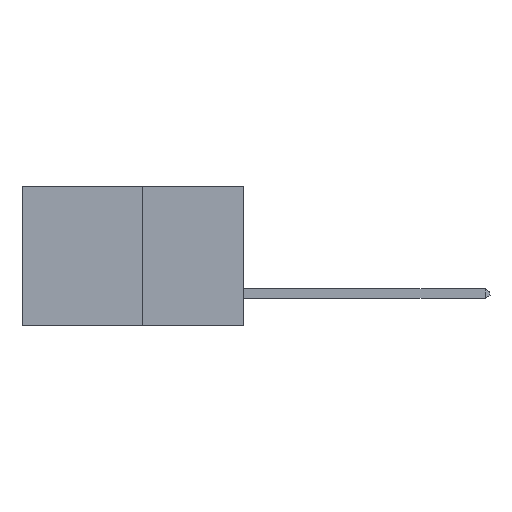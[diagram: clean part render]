
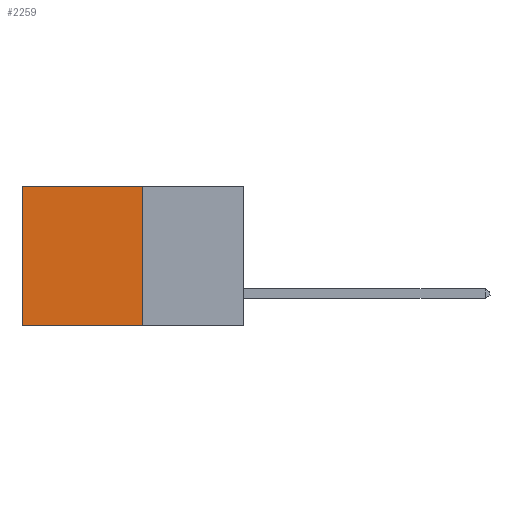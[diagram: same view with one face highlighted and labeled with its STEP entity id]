
A CAD part, left-side view. The second image highlights one B-rep face of the part: STEP entity #2259.
In plain terms, the highlighted planar face has unit normal (-1, 0, 0).
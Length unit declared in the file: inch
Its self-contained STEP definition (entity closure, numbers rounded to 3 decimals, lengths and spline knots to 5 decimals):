
#168 = LINE ( 'NONE', #9690, #10911 ) ;
#216 = VERTEX_POINT ( 'NONE', #3422 ) ;
#265 = EDGE_CURVE ( 'NONE', #3902, #216, #9860, .T. ) ;
#288 = ORIENTED_EDGE ( 'NONE', *, *, #2678, .F. ) ;
#728 = CARTESIAN_POINT ( 'NONE',  ( 0.277, 0.27, -0.37 ) ) ;
#844 = ORIENTED_EDGE ( 'NONE', *, *, #265, .T. ) ;
#880 = DIRECTION ( 'NONE',  ( 0., 1., 0. ) ) ;
#1134 = EDGE_LOOP ( 'NONE', ( #844, #288, #4003, #7695 ) ) ;
#2259 = ADVANCED_FACE ( 'NONE', ( #6381 ), #5868, .F. ) ;
#2678 = EDGE_CURVE ( 'NONE', #2979, #216, #9930, .T. ) ;
#2979 = VERTEX_POINT ( 'NONE', #10078 ) ;
#3100 = VECTOR ( 'NONE', #10730, 39.37008 ) ;
#3422 = CARTESIAN_POINT ( 'NONE',  ( 0.277, 0.59, -0.37 ) ) ;
#3902 = VERTEX_POINT ( 'NONE', #10510 ) ;
#4003 = ORIENTED_EDGE ( 'NONE', *, *, #7244, .F. ) ;
#4107 = VERTEX_POINT ( 'NONE', #10610 ) ;
#5145 = EDGE_CURVE ( 'NONE', #4107, #3902, #7676, .T. ) ;
#5452 = VECTOR ( 'NONE', #8115, 39.37008 ) ;
#5540 = CARTESIAN_POINT ( 'NONE',  ( 0.277, 0.59, -0.37 ) ) ;
#5576 = DIRECTION ( 'NONE',  ( 0., 0., -1. ) ) ;
#5814 = VECTOR ( 'NONE', #880, 39.37008 ) ;
#5868 = PLANE ( 'NONE',  #9458 ) ;
#6083 = CARTESIAN_POINT ( 'NONE',  ( 0.277, 0.27, -0.37 ) ) ;
#6155 = DIRECTION ( 'NONE',  ( 1., 0., 0. ) ) ;
#6381 = FACE_OUTER_BOUND ( 'NONE', #1134, .T. ) ;
#7244 = EDGE_CURVE ( 'NONE', #4107, #2979, #168, .T. ) ;
#7676 = LINE ( 'NONE', #10740, #3100 ) ;
#7695 = ORIENTED_EDGE ( 'NONE', *, *, #5145, .T. ) ;
#8003 = DIRECTION ( 'NONE',  ( 0., 0., -1. ) ) ;
#8115 = DIRECTION ( 'NONE',  ( 0., 0., -1. ) ) ;
#9458 = AXIS2_PLACEMENT_3D ( 'NONE', #6083, #6155, #8003 ) ;
#9690 = CARTESIAN_POINT ( 'NONE',  ( 0.277, 0.27, -0.37 ) ) ;
#9860 = LINE ( 'NONE', #5540, #5452 ) ;
#9930 = LINE ( 'NONE', #728, #5814 ) ;
#10078 = CARTESIAN_POINT ( 'NONE',  ( 0.277, 0.27, -0.37 ) ) ;
#10510 = CARTESIAN_POINT ( 'NONE',  ( 0.277, 0.59, 0. ) ) ;
#10610 = CARTESIAN_POINT ( 'NONE',  ( 0.277, 0.27, 0. ) ) ;
#10730 = DIRECTION ( 'NONE',  ( 0., 1., 0. ) ) ;
#10740 = CARTESIAN_POINT ( 'NONE',  ( 0.277, 0.27, 0. ) ) ;
#10911 = VECTOR ( 'NONE', #5576, 39.37008 ) ;
